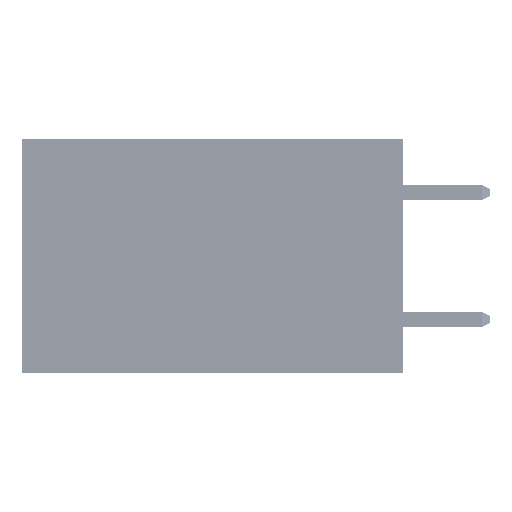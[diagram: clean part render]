
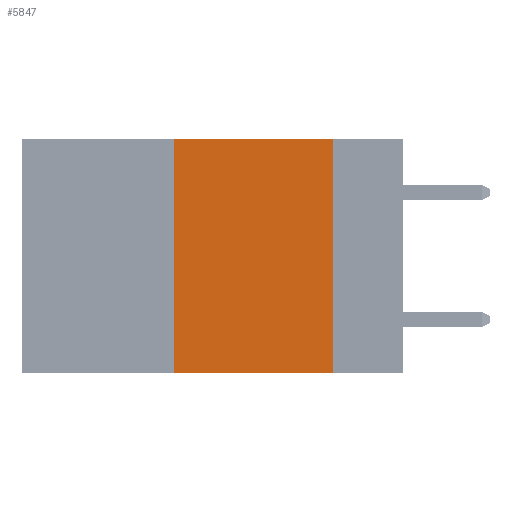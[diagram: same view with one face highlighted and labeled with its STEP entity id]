
A CAD part, left-side view. The second image highlights one B-rep face of the part: STEP entity #5847.
In plain terms, the highlighted planar face has unit normal (-1, 0, 0).
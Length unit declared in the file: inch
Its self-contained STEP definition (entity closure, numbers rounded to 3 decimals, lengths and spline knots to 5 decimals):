
#1827 = LINE ( 'NONE', #42443, #13828 ) ;
#5847 = ADVANCED_FACE ( 'NONE', ( #19030 ), #50518, .F. ) ;
#6498 = CARTESIAN_POINT ( 'NONE',  ( 0., 0.6, 0. ) ) ;
#6601 = VECTOR ( 'NONE', #15007, 39.37008 ) ;
#6762 = DIRECTION ( 'NONE',  ( 1., 0., 0. ) ) ;
#6910 = EDGE_CURVE ( 'NONE', #51677, #49268, #11617, .T. ) ;
#7392 = ORIENTED_EDGE ( 'NONE', *, *, #37643, .F. ) ;
#7892 = CARTESIAN_POINT ( 'NONE',  ( 0., 0.11, 0. ) ) ;
#8405 = LINE ( 'NONE', #7892, #9972 ) ;
#9406 = EDGE_CURVE ( 'NONE', #36629, #14486, #1827, .T. ) ;
#9972 = VECTOR ( 'NONE', #23598, 39.37008 ) ;
#10564 = CARTESIAN_POINT ( 'NONE',  ( 0., 0.36, 0. ) ) ;
#11277 = ORIENTED_EDGE ( 'NONE', *, *, #15493, .F. ) ;
#11617 = LINE ( 'NONE', #31236, #31525 ) ;
#13828 = VECTOR ( 'NONE', #33771, 39.37008 ) ;
#14486 = VERTEX_POINT ( 'NONE', #35107 ) ;
#15007 = DIRECTION ( 'NONE',  ( 0., 0., 1. ) ) ;
#15283 = ORIENTED_EDGE ( 'NONE', *, *, #6910, .F. ) ;
#15493 = EDGE_CURVE ( 'NONE', #36629, #51677, #31232, .T. ) ;
#17196 = CARTESIAN_POINT ( 'NONE',  ( 0., 0.11, 0. ) ) ;
#19030 = FACE_OUTER_BOUND ( 'NONE', #26587, .T. ) ;
#23115 = DIRECTION ( 'NONE',  ( 0., -1., 0. ) ) ;
#23598 = DIRECTION ( 'NONE',  ( 0., 0., -1. ) ) ;
#26154 = CARTESIAN_POINT ( 'NONE',  ( 0., 0.36, -0.37 ) ) ;
#26587 = EDGE_LOOP ( 'NONE', ( #7392, #15283, #11277, #47400 ) ) ;
#29815 = AXIS2_PLACEMENT_3D ( 'NONE', #6498, #6762, #34259 ) ;
#31232 = LINE ( 'NONE', #10564, #6601 ) ;
#31236 = CARTESIAN_POINT ( 'NONE',  ( 0., 0.6, 0. ) ) ;
#31525 = VECTOR ( 'NONE', #23115, 39.37008 ) ;
#33771 = DIRECTION ( 'NONE',  ( 0., -1., 0. ) ) ;
#34259 = DIRECTION ( 'NONE',  ( 0., 0., -1. ) ) ;
#35107 = CARTESIAN_POINT ( 'NONE',  ( 0., 0.11, -0.37 ) ) ;
#36629 = VERTEX_POINT ( 'NONE', #26154 ) ;
#37643 = EDGE_CURVE ( 'NONE', #49268, #14486, #8405, .T. ) ;
#42443 = CARTESIAN_POINT ( 'NONE',  ( 0., 0.6, -0.37 ) ) ;
#47400 = ORIENTED_EDGE ( 'NONE', *, *, #9406, .T. ) ;
#47653 = CARTESIAN_POINT ( 'NONE',  ( 0., 0.36, 0. ) ) ;
#49268 = VERTEX_POINT ( 'NONE', #17196 ) ;
#50518 = PLANE ( 'NONE',  #29815 ) ;
#51677 = VERTEX_POINT ( 'NONE', #47653 ) ;
